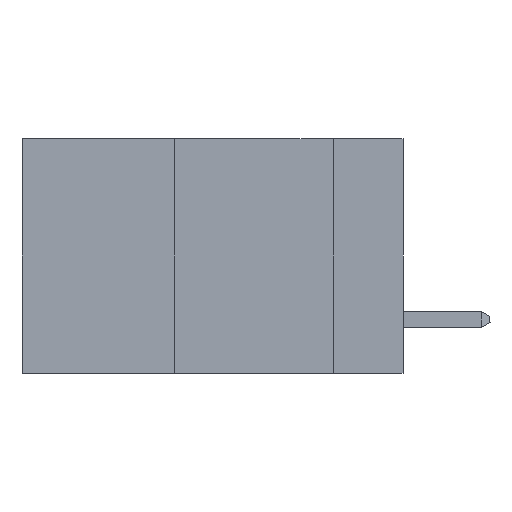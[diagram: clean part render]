
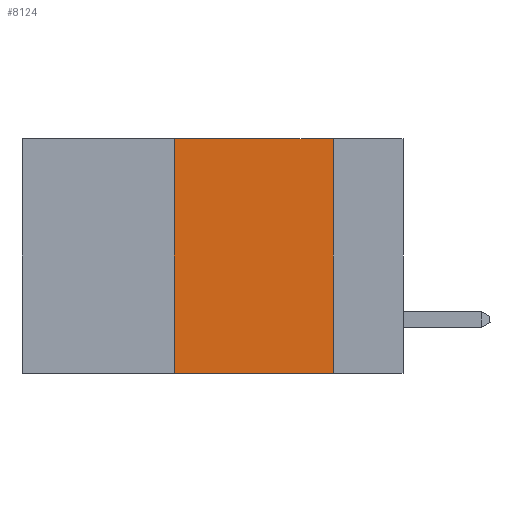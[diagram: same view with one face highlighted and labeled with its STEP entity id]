
A CAD part, left-side view. The second image highlights one B-rep face of the part: STEP entity #8124.
In plain terms, the highlighted planar face has unit normal (-1, 0, 0).
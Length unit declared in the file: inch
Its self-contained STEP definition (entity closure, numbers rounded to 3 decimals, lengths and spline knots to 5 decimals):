
#609 = DIRECTION ( 'NONE',  ( 0., 0., -1. ) ) ;
#1527 = EDGE_CURVE ( 'NONE', #12512, #10427, #1781, .T. ) ;
#1781 = LINE ( 'NONE', #15201, #13638 ) ;
#1947 = DIRECTION ( 'NONE',  ( 0., -1., 0. ) ) ;
#2497 = ORIENTED_EDGE ( 'NONE', *, *, #4293, .F. ) ;
#3616 = ORIENTED_EDGE ( 'NONE', *, *, #11878, .T. ) ;
#4079 = VERTEX_POINT ( 'NONE', #14218 ) ;
#4097 = DIRECTION ( 'NONE',  ( 0., -1., 0. ) ) ;
#4293 = EDGE_CURVE ( 'NONE', #18231, #4079, #19234, .T. ) ;
#4493 = CARTESIAN_POINT ( 'NONE',  ( 0., 0.11, 0. ) ) ;
#4573 = ORIENTED_EDGE ( 'NONE', *, *, #1527, .F. ) ;
#5181 = EDGE_CURVE ( 'NONE', #10427, #18231, #16307, .T. ) ;
#5421 = CARTESIAN_POINT ( 'NONE',  ( 0., 0.6, 0. ) ) ;
#6647 = VECTOR ( 'NONE', #609, 39.37008 ) ;
#6750 = CARTESIAN_POINT ( 'NONE',  ( 0., 0.36, 0. ) ) ;
#7145 = AXIS2_PLACEMENT_3D ( 'NONE', #17155, #12864, #17632 ) ;
#8124 = ADVANCED_FACE ( 'NONE', ( #18137 ), #12537, .F. ) ;
#9043 = VECTOR ( 'NONE', #1947, 39.37008 ) ;
#10427 = VERTEX_POINT ( 'NONE', #6750 ) ;
#11743 = VECTOR ( 'NONE', #4097, 39.37008 ) ;
#11878 = EDGE_CURVE ( 'NONE', #12512, #4079, #14846, .T. ) ;
#12447 = CARTESIAN_POINT ( 'NONE',  ( 0., 0.36, -0.37 ) ) ;
#12512 = VERTEX_POINT ( 'NONE', #12447 ) ;
#12537 = PLANE ( 'NONE',  #7145 ) ;
#12864 = DIRECTION ( 'NONE',  ( 1., 0., 0. ) ) ;
#13638 = VECTOR ( 'NONE', #15139, 39.37008 ) ;
#14138 = EDGE_LOOP ( 'NONE', ( #2497, #15554, #4573, #3616 ) ) ;
#14218 = CARTESIAN_POINT ( 'NONE',  ( 0., 0.11, -0.37 ) ) ;
#14558 = CARTESIAN_POINT ( 'NONE',  ( 0., 0.11, 0. ) ) ;
#14846 = LINE ( 'NONE', #15728, #9043 ) ;
#15139 = DIRECTION ( 'NONE',  ( 0., 0., 1. ) ) ;
#15201 = CARTESIAN_POINT ( 'NONE',  ( 0., 0.36, 0. ) ) ;
#15554 = ORIENTED_EDGE ( 'NONE', *, *, #5181, .F. ) ;
#15728 = CARTESIAN_POINT ( 'NONE',  ( 0., 0.6, -0.37 ) ) ;
#16307 = LINE ( 'NONE', #5421, #11743 ) ;
#17155 = CARTESIAN_POINT ( 'NONE',  ( 0., 0.6, 0. ) ) ;
#17632 = DIRECTION ( 'NONE',  ( 0., 0., -1. ) ) ;
#18137 = FACE_OUTER_BOUND ( 'NONE', #14138, .T. ) ;
#18231 = VERTEX_POINT ( 'NONE', #4493 ) ;
#19234 = LINE ( 'NONE', #14558, #6647 ) ;
